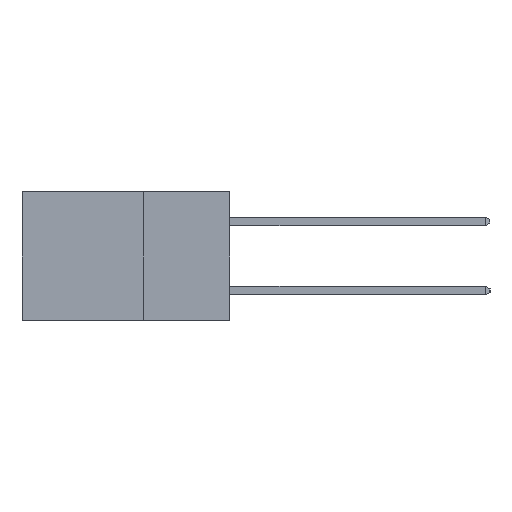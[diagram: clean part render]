
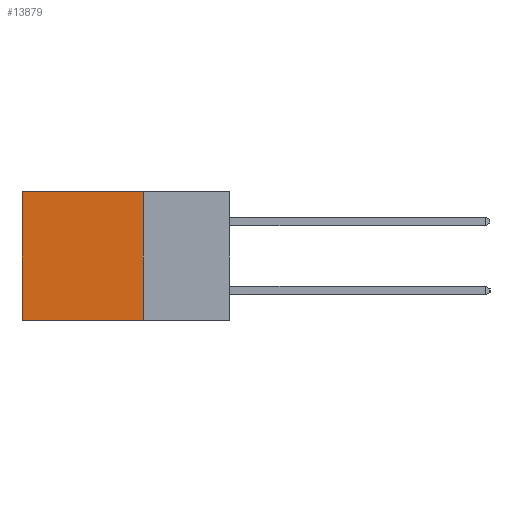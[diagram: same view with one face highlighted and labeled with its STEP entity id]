
A CAD part, left-side view. The second image highlights one B-rep face of the part: STEP entity #13879.
In plain terms, the highlighted planar face has unit normal (-1, 0, 0).
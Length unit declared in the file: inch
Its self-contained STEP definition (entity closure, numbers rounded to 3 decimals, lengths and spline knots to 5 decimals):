
#327 = DIRECTION ( 'NONE',  ( 1., 0., 0. ) ) ;
#952 = CARTESIAN_POINT ( 'NONE',  ( 0.2615, 0.25, -0.37 ) ) ;
#1017 = VECTOR ( 'NONE', #12387, 39.37008 ) ;
#1728 = CARTESIAN_POINT ( 'NONE',  ( 0.2615, 0.25, -0.37 ) ) ;
#1946 = VECTOR ( 'NONE', #11602, 39.37008 ) ;
#2805 = EDGE_CURVE ( 'NONE', #15464, #13925, #5524, .T. ) ;
#3181 = CARTESIAN_POINT ( 'NONE',  ( 0.2615, 0.6, 0. ) ) ;
#3311 = VERTEX_POINT ( 'NONE', #5808 ) ;
#3578 = EDGE_CURVE ( 'NONE', #15464, #9241, #14199, .T. ) ;
#4163 = ORIENTED_EDGE ( 'NONE', *, *, #5938, .F. ) ;
#4636 = LINE ( 'NONE', #1728, #1017 ) ;
#4665 = DIRECTION ( 'NONE',  ( 0., 0., -1. ) ) ;
#5524 = LINE ( 'NONE', #8438, #1946 ) ;
#5798 = ORIENTED_EDGE ( 'NONE', *, *, #6476, .T. ) ;
#5808 = CARTESIAN_POINT ( 'NONE',  ( 0.2615, 0.6, -0.37 ) ) ;
#5938 = EDGE_CURVE ( 'NONE', #9241, #3311, #4636, .T. ) ;
#6460 = LINE ( 'NONE', #12588, #13103 ) ;
#6476 = EDGE_CURVE ( 'NONE', #13925, #3311, #6460, .T. ) ;
#8102 = CARTESIAN_POINT ( 'NONE',  ( 0.2615, 0.25, -0.37 ) ) ;
#8208 = EDGE_LOOP ( 'NONE', ( #5798, #4163, #8348, #17005 ) ) ;
#8348 = ORIENTED_EDGE ( 'NONE', *, *, #3578, .F. ) ;
#8438 = CARTESIAN_POINT ( 'NONE',  ( 0.2615, 0.25, 0. ) ) ;
#9241 = VERTEX_POINT ( 'NONE', #8102 ) ;
#9698 = DIRECTION ( 'NONE',  ( 0., 0., -1. ) ) ;
#10667 = VECTOR ( 'NONE', #11665, 39.37008 ) ;
#11602 = DIRECTION ( 'NONE',  ( 0., 1., 0. ) ) ;
#11665 = DIRECTION ( 'NONE',  ( 0., 0., -1. ) ) ;
#12387 = DIRECTION ( 'NONE',  ( 0., 1., 0. ) ) ;
#12588 = CARTESIAN_POINT ( 'NONE',  ( 0.2615, 0.6, -0.37 ) ) ;
#13103 = VECTOR ( 'NONE', #4665, 39.37008 ) ;
#13879 = ADVANCED_FACE ( 'NONE', ( #14094 ), #16294, .F. ) ;
#13925 = VERTEX_POINT ( 'NONE', #3181 ) ;
#14094 = FACE_OUTER_BOUND ( 'NONE', #8208, .T. ) ;
#14199 = LINE ( 'NONE', #952, #10667 ) ;
#14971 = CARTESIAN_POINT ( 'NONE',  ( 0.2615, 0.25, -0.37 ) ) ;
#15464 = VERTEX_POINT ( 'NONE', #16919 ) ;
#16294 = PLANE ( 'NONE',  #16349 ) ;
#16349 = AXIS2_PLACEMENT_3D ( 'NONE', #14971, #327, #9698 ) ;
#16919 = CARTESIAN_POINT ( 'NONE',  ( 0.2615, 0.25, 0. ) ) ;
#17005 = ORIENTED_EDGE ( 'NONE', *, *, #2805, .T. ) ;
